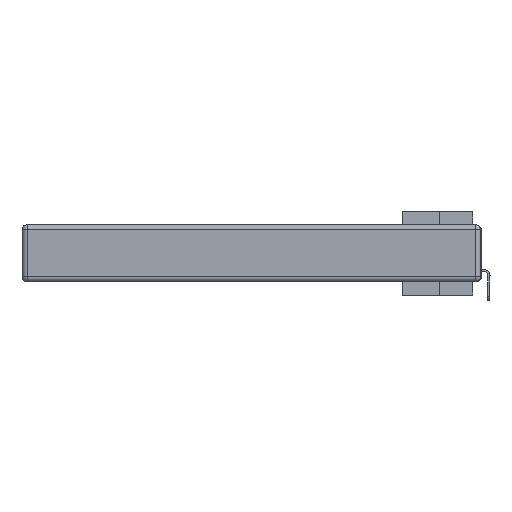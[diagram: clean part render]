
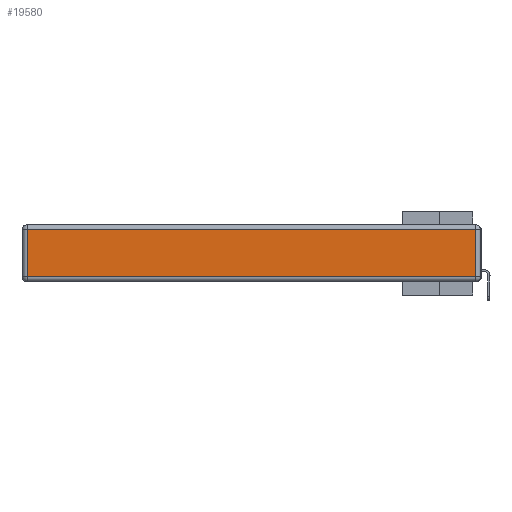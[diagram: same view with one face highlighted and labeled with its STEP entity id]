
A CAD part, left-side view. The second image highlights one B-rep face of the part: STEP entity #19580.
In plain terms, the highlighted planar face has unit normal (-1, 0, 0).
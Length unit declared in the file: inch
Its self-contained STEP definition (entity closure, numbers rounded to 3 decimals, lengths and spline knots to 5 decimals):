
#535 = CARTESIAN_POINT ( 'NONE',  ( 0., 2.75, -0.03 ) ) ;
#1310 = EDGE_CURVE ( 'NONE', #12557, #14100, #3278, .T. ) ;
#2069 = FACE_OUTER_BOUND ( 'NONE', #17231, .T. ) ;
#2743 = ORIENTED_EDGE ( 'NONE', *, *, #1310, .T. ) ;
#3278 = LINE ( 'NONE', #535, #29216 ) ;
#3785 = CARTESIAN_POINT ( 'NONE',  ( 0., 0.03, -0.03 ) ) ;
#5182 = ORIENTED_EDGE ( 'NONE', *, *, #14308, .T. ) ;
#5769 = DIRECTION ( 'NONE',  ( 0., -1., 0. ) ) ;
#8908 = EDGE_CURVE ( 'NONE', #9491, #15748, #33778, .T. ) ;
#9491 = VERTEX_POINT ( 'NONE', #12259 ) ;
#10174 = ORIENTED_EDGE ( 'NONE', *, *, #8908, .T. ) ;
#10896 = CARTESIAN_POINT ( 'NONE',  ( 0., 2.72, -0.343 ) ) ;
#12259 = CARTESIAN_POINT ( 'NONE',  ( 0., 2.72, -0.313 ) ) ;
#12557 = VERTEX_POINT ( 'NONE', #3785 ) ;
#14100 = VERTEX_POINT ( 'NONE', #15282 ) ;
#14308 = EDGE_CURVE ( 'NONE', #14100, #9491, #28651, .T. ) ;
#14516 = DIRECTION ( 'NONE',  ( 0., 1., 0. ) ) ;
#15282 = CARTESIAN_POINT ( 'NONE',  ( 0., 2.72, -0.03 ) ) ;
#15482 = EDGE_CURVE ( 'NONE', #15748, #12557, #18394, .T. ) ;
#15595 = AXIS2_PLACEMENT_3D ( 'NONE', #29869, #20960, #18062 ) ;
#15748 = VERTEX_POINT ( 'NONE', #19806 ) ;
#16304 = VECTOR ( 'NONE', #16537, 39.37008 ) ;
#16537 = DIRECTION ( 'NONE',  ( 0., 0., -1. ) ) ;
#17231 = EDGE_LOOP ( 'NONE', ( #10174, #29603, #2743, #5182 ) ) ;
#18062 = DIRECTION ( 'NONE',  ( 0., 0., 1. ) ) ;
#18219 = CARTESIAN_POINT ( 'NONE',  ( 0., 0.03, -0.343 ) ) ;
#18394 = LINE ( 'NONE', #18219, #24634 ) ;
#18919 = VECTOR ( 'NONE', #5769, 39.37008 ) ;
#19580 = ADVANCED_FACE ( 'NONE', ( #2069 ), #35164, .T. ) ;
#19806 = CARTESIAN_POINT ( 'NONE',  ( 0., 0.03, -0.313 ) ) ;
#20960 = DIRECTION ( 'NONE',  ( -1., 0., 0. ) ) ;
#24634 = VECTOR ( 'NONE', #34607, 39.37008 ) ;
#28651 = LINE ( 'NONE', #10896, #16304 ) ;
#29216 = VECTOR ( 'NONE', #14516, 39.37008 ) ;
#29603 = ORIENTED_EDGE ( 'NONE', *, *, #15482, .T. ) ;
#29869 = CARTESIAN_POINT ( 'NONE',  ( 0., 0., -0.343 ) ) ;
#30502 = CARTESIAN_POINT ( 'NONE',  ( 0., 0., -0.313 ) ) ;
#33778 = LINE ( 'NONE', #30502, #18919 ) ;
#34607 = DIRECTION ( 'NONE',  ( 0., 0., 1. ) ) ;
#35164 = PLANE ( 'NONE',  #15595 ) ;
